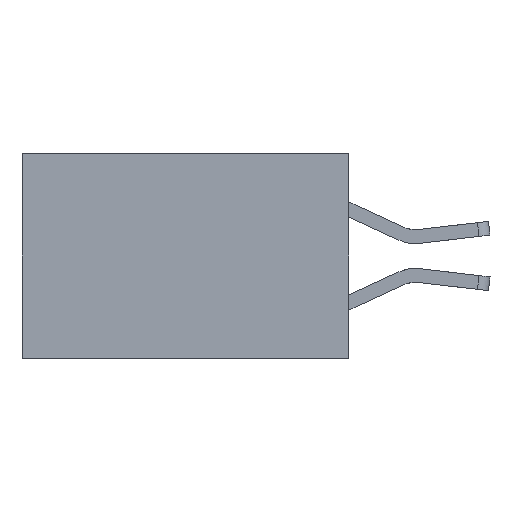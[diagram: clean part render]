
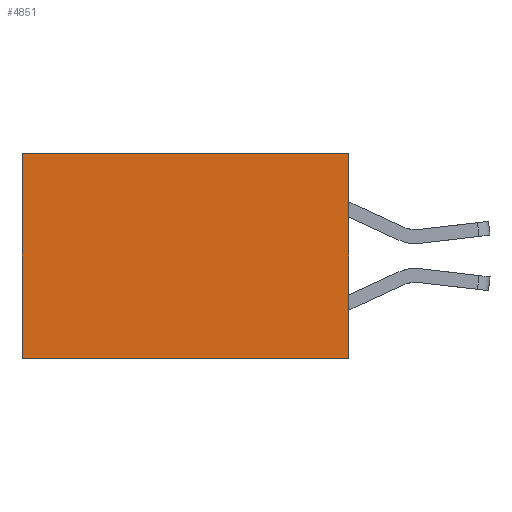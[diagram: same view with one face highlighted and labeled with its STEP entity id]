
A CAD part, left-side view. The second image highlights one B-rep face of the part: STEP entity #4851.
In plain terms, the highlighted planar face has unit normal (-1, 0, 0).
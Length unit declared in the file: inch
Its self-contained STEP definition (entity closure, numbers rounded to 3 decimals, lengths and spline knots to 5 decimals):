
#523 = CARTESIAN_POINT ( 'NONE',  ( 0.277, 0., 0. ) ) ;
#631 = ORIENTED_EDGE ( 'NONE', *, *, #2486, .F. ) ;
#639 = ORIENTED_EDGE ( 'NONE', *, *, #3360, .T. ) ;
#1011 = ORIENTED_EDGE ( 'NONE', *, *, #9367, .T. ) ;
#1073 = VERTEX_POINT ( 'NONE', #7725 ) ;
#1396 = LINE ( 'NONE', #8591, #1645 ) ;
#1645 = VECTOR ( 'NONE', #5088, 39.37008 ) ;
#2084 = CARTESIAN_POINT ( 'NONE',  ( 0.277, 0.59, -0.37 ) ) ;
#2340 = EDGE_LOOP ( 'NONE', ( #1011, #631, #6563, #639 ) ) ;
#2422 = AXIS2_PLACEMENT_3D ( 'NONE', #8381, #8528, #8984 ) ;
#2486 = EDGE_CURVE ( 'NONE', #7529, #10054, #1396, .T. ) ;
#3360 = EDGE_CURVE ( 'NONE', #6840, #1073, #8657, .T. ) ;
#3371 = VECTOR ( 'NONE', #7801, 39.37008 ) ;
#4406 = VECTOR ( 'NONE', #9891, 39.37008 ) ;
#4851 = ADVANCED_FACE ( 'NONE', ( #10115 ), #8505, .F. ) ;
#4972 = LINE ( 'NONE', #6774, #8962 ) ;
#5088 = DIRECTION ( 'NONE',  ( 0., 1., 0. ) ) ;
#5963 = CARTESIAN_POINT ( 'NONE',  ( 0.277, 0., -0.37 ) ) ;
#6563 = ORIENTED_EDGE ( 'NONE', *, *, #7222, .F. ) ;
#6699 = DIRECTION ( 'NONE',  ( 0., 0., -1. ) ) ;
#6774 = CARTESIAN_POINT ( 'NONE',  ( 0.277, 0.59, -0.37 ) ) ;
#6840 = VERTEX_POINT ( 'NONE', #523 ) ;
#7222 = EDGE_CURVE ( 'NONE', #6840, #7529, #7671, .T. ) ;
#7529 = VERTEX_POINT ( 'NONE', #5963 ) ;
#7671 = LINE ( 'NONE', #7832, #3371 ) ;
#7725 = CARTESIAN_POINT ( 'NONE',  ( 0.277, 0.59, 0. ) ) ;
#7801 = DIRECTION ( 'NONE',  ( 0., 0., -1. ) ) ;
#7832 = CARTESIAN_POINT ( 'NONE',  ( 0.277, 0., -0.37 ) ) ;
#8381 = CARTESIAN_POINT ( 'NONE',  ( 0.277, 0., -0.37 ) ) ;
#8505 = PLANE ( 'NONE',  #2422 ) ;
#8528 = DIRECTION ( 'NONE',  ( 1., 0., 0. ) ) ;
#8591 = CARTESIAN_POINT ( 'NONE',  ( 0.277, 0., -0.37 ) ) ;
#8657 = LINE ( 'NONE', #9954, #4406 ) ;
#8962 = VECTOR ( 'NONE', #6699, 39.37008 ) ;
#8984 = DIRECTION ( 'NONE',  ( 0., 0., -1. ) ) ;
#9367 = EDGE_CURVE ( 'NONE', #1073, #10054, #4972, .T. ) ;
#9891 = DIRECTION ( 'NONE',  ( 0., 1., 0. ) ) ;
#9954 = CARTESIAN_POINT ( 'NONE',  ( 0.277, 0., 0. ) ) ;
#10054 = VERTEX_POINT ( 'NONE', #2084 ) ;
#10115 = FACE_OUTER_BOUND ( 'NONE', #2340, .T. ) ;
